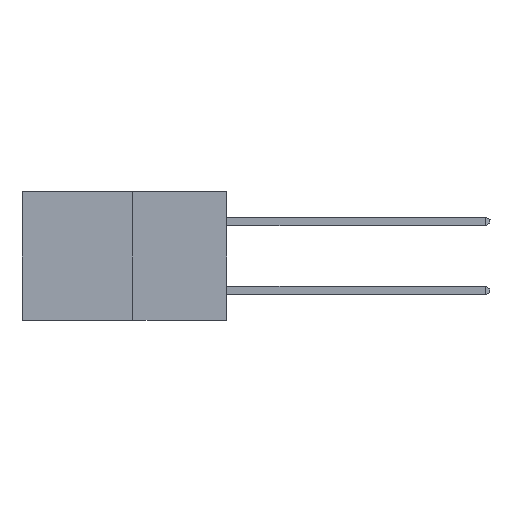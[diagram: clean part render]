
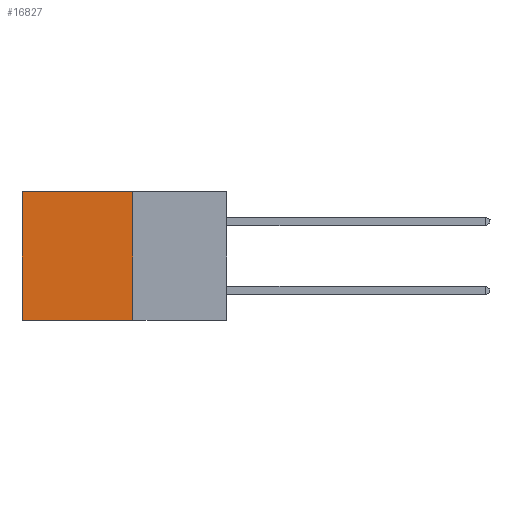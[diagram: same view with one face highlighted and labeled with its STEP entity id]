
A CAD part, left-side view. The second image highlights one B-rep face of the part: STEP entity #16827.
In plain terms, the highlighted planar face has unit normal (-1, 0, 0).
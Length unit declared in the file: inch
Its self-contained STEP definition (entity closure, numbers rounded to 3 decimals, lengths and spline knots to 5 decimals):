
#399 = ORIENTED_EDGE ( 'NONE', *, *, #22725, .T. ) ;
#2466 = LINE ( 'NONE', #26127, #14710 ) ;
#3534 = CARTESIAN_POINT ( 'NONE',  ( 0.277, 0.27, -0.37 ) ) ;
#4601 = LINE ( 'NONE', #22319, #28908 ) ;
#4746 = CARTESIAN_POINT ( 'NONE',  ( 0.277, 0.27, -0.37 ) ) ;
#5203 = DIRECTION ( 'NONE',  ( 0., 1., 0. ) ) ;
#6196 = VERTEX_POINT ( 'NONE', #3534 ) ;
#6600 = VERTEX_POINT ( 'NONE', #12282 ) ;
#7096 = EDGE_LOOP ( 'NONE', ( #399, #9073, #31392, #16719 ) ) ;
#7234 = DIRECTION ( 'NONE',  ( 0., 0., -1. ) ) ;
#7427 = DIRECTION ( 'NONE',  ( 0., 1., 0. ) ) ;
#7945 = FACE_OUTER_BOUND ( 'NONE', #7096, .T. ) ;
#9073 = ORIENTED_EDGE ( 'NONE', *, *, #9432, .F. ) ;
#9432 = EDGE_CURVE ( 'NONE', #6196, #6600, #31139, .T. ) ;
#9613 = CARTESIAN_POINT ( 'NONE',  ( 0.277, 0.59, 0. ) ) ;
#11619 = DIRECTION ( 'NONE',  ( 0., 0., -1. ) ) ;
#12282 = CARTESIAN_POINT ( 'NONE',  ( 0.277, 0.59, -0.37 ) ) ;
#12344 = CARTESIAN_POINT ( 'NONE',  ( 0.277, 0.27, 0. ) ) ;
#12372 = CARTESIAN_POINT ( 'NONE',  ( 0.277, 0.27, -0.37 ) ) ;
#14710 = VECTOR ( 'NONE', #11619, 39.37008 ) ;
#15613 = VERTEX_POINT ( 'NONE', #12344 ) ;
#15639 = LINE ( 'NONE', #29053, #27709 ) ;
#16251 = VERTEX_POINT ( 'NONE', #9613 ) ;
#16719 = ORIENTED_EDGE ( 'NONE', *, *, #31146, .T. ) ;
#16827 = ADVANCED_FACE ( 'NONE', ( #7945 ), #23752, .F. ) ;
#17069 = DIRECTION ( 'NONE',  ( 0., 0., -1. ) ) ;
#21878 = DIRECTION ( 'NONE',  ( 1., 0., 0. ) ) ;
#22319 = CARTESIAN_POINT ( 'NONE',  ( 0.277, 0.27, 0. ) ) ;
#22725 = EDGE_CURVE ( 'NONE', #16251, #6600, #15639, .T. ) ;
#23752 = PLANE ( 'NONE',  #23828 ) ;
#23828 = AXIS2_PLACEMENT_3D ( 'NONE', #4746, #21878, #7234 ) ;
#24027 = VECTOR ( 'NONE', #7427, 39.37008 ) ;
#24951 = EDGE_CURVE ( 'NONE', #15613, #6196, #2466, .T. ) ;
#26127 = CARTESIAN_POINT ( 'NONE',  ( 0.277, 0.27, -0.37 ) ) ;
#27709 = VECTOR ( 'NONE', #17069, 39.37008 ) ;
#28908 = VECTOR ( 'NONE', #5203, 39.37008 ) ;
#29053 = CARTESIAN_POINT ( 'NONE',  ( 0.277, 0.59, -0.37 ) ) ;
#31139 = LINE ( 'NONE', #12372, #24027 ) ;
#31146 = EDGE_CURVE ( 'NONE', #15613, #16251, #4601, .T. ) ;
#31392 = ORIENTED_EDGE ( 'NONE', *, *, #24951, .F. ) ;
